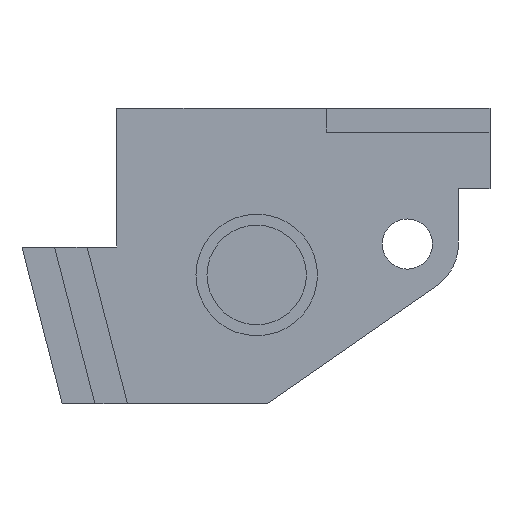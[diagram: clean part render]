
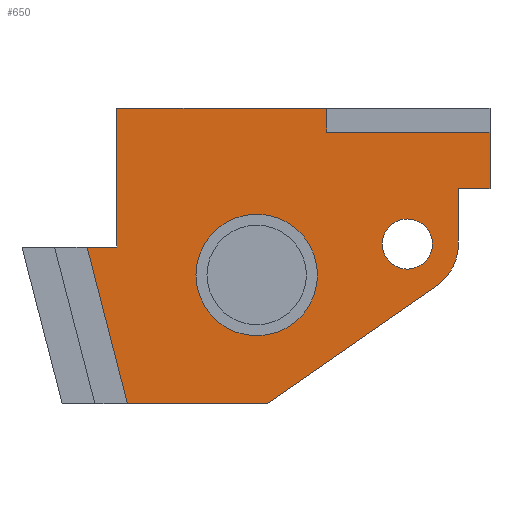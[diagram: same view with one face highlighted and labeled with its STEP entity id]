
A CAD part, left-side view. The second image highlights one B-rep face of the part: STEP entity #650.
In plain terms, the highlighted planar face has unit normal (-1, 0, 0).
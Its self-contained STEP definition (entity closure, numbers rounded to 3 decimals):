
#16=FACE_BOUND('',#90,.T.);
#17=FACE_BOUND('',#91,.T.);
#20=PLANE('',#703);
#53=FACE_OUTER_BOUND('',#89,.T.);
#89=EDGE_LOOP('',(#467,#468,#469,#470,#471,#472,#473,#474,#475,#476,#477,
#478));
#90=EDGE_LOOP('',(#479));
#91=EDGE_LOOP('',(#480));
#126=LINE('',#929,#211);
#127=LINE('',#931,#212);
#128=LINE('',#933,#213);
#129=LINE('',#937,#214);
#130=LINE('',#939,#215);
#131=LINE('',#941,#216);
#132=LINE('',#943,#217);
#133=LINE('',#945,#218);
#134=LINE('',#947,#219);
#135=LINE('',#949,#220);
#136=LINE('',#950,#221);
#211=VECTOR('',#759,10.);
#212=VECTOR('',#760,10.);
#213=VECTOR('',#761,10.);
#214=VECTOR('',#764,10.);
#215=VECTOR('',#765,10.);
#216=VECTOR('',#766,10.);
#217=VECTOR('',#767,10.);
#218=VECTOR('',#768,10.);
#219=VECTOR('',#769,10.);
#220=VECTOR('',#770,10.);
#221=VECTOR('',#771,10.);
#297=CIRCLE('',#701,3.85);
#298=CIRCLE('',#704,3.24);
#299=CIRCLE('',#705,1.59);
#305=VERTEX_POINT('',#922);
#306=VERTEX_POINT('',#927);
#307=VERTEX_POINT('',#928);
#308=VERTEX_POINT('',#930);
#309=VERTEX_POINT('',#932);
#310=VERTEX_POINT('',#934);
#311=VERTEX_POINT('',#936);
#312=VERTEX_POINT('',#938);
#313=VERTEX_POINT('',#940);
#314=VERTEX_POINT('',#942);
#315=VERTEX_POINT('',#944);
#316=VERTEX_POINT('',#946);
#317=VERTEX_POINT('',#948);
#318=VERTEX_POINT('',#951);
#369=EDGE_CURVE('',#305,#305,#297,.T.);
#370=EDGE_CURVE('',#306,#307,#126,.T.);
#371=EDGE_CURVE('',#307,#308,#127,.T.);
#372=EDGE_CURVE('',#308,#309,#128,.T.);
#373=EDGE_CURVE('',#310,#309,#298,.T.);
#374=EDGE_CURVE('',#311,#310,#129,.T.);
#375=EDGE_CURVE('',#311,#312,#130,.T.);
#376=EDGE_CURVE('',#312,#313,#131,.T.);
#377=EDGE_CURVE('',#313,#314,#132,.T.);
#378=EDGE_CURVE('',#314,#315,#133,.T.);
#379=EDGE_CURVE('',#316,#315,#134,.T.);
#380=EDGE_CURVE('',#316,#317,#135,.T.);
#381=EDGE_CURVE('',#317,#306,#136,.T.);
#382=EDGE_CURVE('',#318,#318,#299,.T.);
#467=ORIENTED_EDGE('',*,*,#370,.T.);
#468=ORIENTED_EDGE('',*,*,#371,.T.);
#469=ORIENTED_EDGE('',*,*,#372,.T.);
#470=ORIENTED_EDGE('',*,*,#373,.F.);
#471=ORIENTED_EDGE('',*,*,#374,.F.);
#472=ORIENTED_EDGE('',*,*,#375,.T.);
#473=ORIENTED_EDGE('',*,*,#376,.T.);
#474=ORIENTED_EDGE('',*,*,#377,.T.);
#475=ORIENTED_EDGE('',*,*,#378,.T.);
#476=ORIENTED_EDGE('',*,*,#379,.F.);
#477=ORIENTED_EDGE('',*,*,#380,.T.);
#478=ORIENTED_EDGE('',*,*,#381,.T.);
#479=ORIENTED_EDGE('',*,*,#382,.F.);
#480=ORIENTED_EDGE('',*,*,#369,.T.);
#650=ADVANCED_FACE('',(#53,#16,#17),#20,.F.);
#701=AXIS2_PLACEMENT_3D('',#924,#753,#754);
#703=AXIS2_PLACEMENT_3D('',#926,#757,#758);
#704=AXIS2_PLACEMENT_3D('',#935,#762,#763);
#705=AXIS2_PLACEMENT_3D('',#952,#772,#773);
#753=DIRECTION('center_axis',(1.,0.,0.));
#754=DIRECTION('ref_axis',(0.,-1.,0.));
#757=DIRECTION('center_axis',(1.,0.,0.));
#758=DIRECTION('ref_axis',(0.,1.,0.));
#759=DIRECTION('',(0.,-0.249,-0.969));
#760=DIRECTION('',(0.,-1.,0.));
#761=DIRECTION('',(0.,-0.821,0.571));
#762=DIRECTION('center_axis',(1.,0.,0.));
#763=DIRECTION('ref_axis',(0.,1.,0.));
#764=DIRECTION('',(0.,0.,-1.));
#765=DIRECTION('',(0.,-1.,0.));
#766=DIRECTION('',(0.,0.,1.));
#767=DIRECTION('',(0.,1.,0.));
#768=DIRECTION('',(0.,0.,1.));
#769=DIRECTION('',(0.,-1.,0.));
#770=DIRECTION('',(0.,0.,-1.));
#771=DIRECTION('',(0.,1.,0.));
#772=DIRECTION('center_axis',(-1.,0.,0.));
#773=DIRECTION('ref_axis',(0.,1.,0.));
#922=CARTESIAN_POINT('',(0.,13.391,-1.96));
#924=CARTESIAN_POINT('Origin',(0.,9.541,-1.96));
#926=CARTESIAN_POINT('Origin',(0.,9.585,-0.76));
#927=CARTESIAN_POINT('',(0.,20.28,-0.19));
#928=CARTESIAN_POINT('',(0.,17.73,-10.11));
#929=CARTESIAN_POINT('',(0.,18.605,-6.707));
#930=CARTESIAN_POINT('',(0.,8.86,-10.11));
#931=CARTESIAN_POINT('',(0.,21.86,-10.11));
#932=CARTESIAN_POINT('',(0.,-1.85,-2.66));
#933=CARTESIAN_POINT('',(0.,8.86,-10.11));
#934=CARTESIAN_POINT('',(0.,-3.24,0.));
#935=CARTESIAN_POINT('Origin',(0.,0.,0.));
#936=CARTESIAN_POINT('',(0.,-3.24,3.49));
#937=CARTESIAN_POINT('',(0.,-3.24,3.49));
#938=CARTESIAN_POINT('',(0.,-5.24,3.49));
#939=CARTESIAN_POINT('',(0.,-3.24,3.49));
#940=CARTESIAN_POINT('',(0.,-5.24,7.09));
#941=CARTESIAN_POINT('',(0.,-5.24,3.49));
#942=CARTESIAN_POINT('',(0.,5.11,7.09));
#943=CARTESIAN_POINT('',(0.,7.348,7.09));
#944=CARTESIAN_POINT('',(0.,5.11,8.59));
#945=CARTESIAN_POINT('',(0.,5.11,3.915));
#946=CARTESIAN_POINT('',(0.,18.41,8.59));
#947=CARTESIAN_POINT('',(0.,18.41,8.59));
#948=CARTESIAN_POINT('',(0.,18.41,-0.19));
#949=CARTESIAN_POINT('',(0.,18.41,8.59));
#950=CARTESIAN_POINT('',(0.,18.41,-0.19));
#951=CARTESIAN_POINT('',(0.,-1.59,0.));
#952=CARTESIAN_POINT('Origin',(0.,0.,0.));
